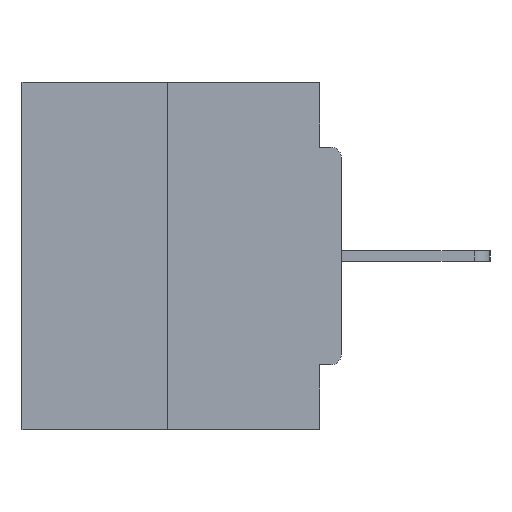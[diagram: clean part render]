
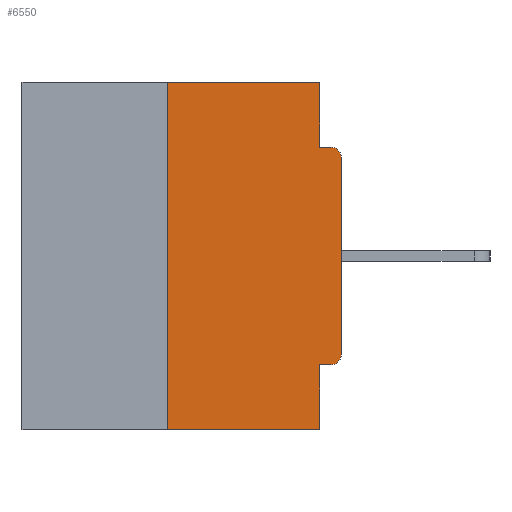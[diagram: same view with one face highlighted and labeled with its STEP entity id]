
A CAD part, left-side view. The second image highlights one B-rep face of the part: STEP entity #6550.
In plain terms, the highlighted planar face has unit normal (-1, 0, 0).
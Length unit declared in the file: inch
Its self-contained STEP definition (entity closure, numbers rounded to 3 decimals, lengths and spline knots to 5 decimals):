
#175 = ORIENTED_EDGE ( 'NONE', *, *, #31595, .F. ) ;
#644 = CARTESIAN_POINT ( 'NONE',  ( 0., 0.031, 0. ) ) ;
#915 = CARTESIAN_POINT ( 'NONE',  ( 0., 0., -0.4065 ) ) ;
#1305 = VERTEX_POINT ( 'NONE', #25709 ) ;
#1580 = DIRECTION ( 'NONE',  ( 0., -1., 0. ) ) ;
#2088 = CARTESIAN_POINT ( 'NONE',  ( 0., 0.031, 0. ) ) ;
#2983 = ORIENTED_EDGE ( 'NONE', *, *, #23573, .F. ) ;
#3215 = EDGE_CURVE ( 'NONE', #24187, #14221, #26456, .T. ) ;
#3456 = VERTEX_POINT ( 'NONE', #5786 ) ;
#3490 = VECTOR ( 'NONE', #1580, 39.37008 ) ;
#3898 = CARTESIAN_POINT ( 'NONE',  ( 0., 0.015, -0.3915 ) ) ;
#3911 = ORIENTED_EDGE ( 'NONE', *, *, #20447, .T. ) ;
#4279 = DIRECTION ( 'NONE',  ( 0., 0., 1. ) ) ;
#4697 = LINE ( 'NONE', #24977, #11802 ) ;
#4890 = EDGE_LOOP ( 'NONE', ( #21691, #175, #27476, #16226, #2983, #3911, #17752, #12775, #15443, #9832 ) ) ;
#5073 = CARTESIAN_POINT ( 'NONE',  ( 0., 0.46, -0.5 ) ) ;
#5786 = CARTESIAN_POINT ( 'NONE',  ( 0., 0.031, -0.0935 ) ) ;
#5982 = LINE ( 'NONE', #6297, #25181 ) ;
#6297 = CARTESIAN_POINT ( 'NONE',  ( 0., 0., 0. ) ) ;
#6550 = ADVANCED_FACE ( 'NONE', ( #20628 ), #17997, .F. ) ;
#7483 = VERTEX_POINT ( 'NONE', #8273 ) ;
#8273 = CARTESIAN_POINT ( 'NONE',  ( 0., 0.25, -0.5 ) ) ;
#8422 = DIRECTION ( 'NONE',  ( 0., 1., 0. ) ) ;
#9832 = ORIENTED_EDGE ( 'NONE', *, *, #13114, .F. ) ;
#9934 = DIRECTION ( 'NONE',  ( 0., -1., 0. ) ) ;
#10700 = AXIS2_PLACEMENT_3D ( 'NONE', #14716, #11786, #19805 ) ;
#10966 = CARTESIAN_POINT ( 'NONE',  ( 0., 0.031, -0.5 ) ) ;
#11416 = DIRECTION ( 'NONE',  ( 0., 0., -1. ) ) ;
#11463 = VECTOR ( 'NONE', #16499, 39.37008 ) ;
#11465 = AXIS2_PLACEMENT_3D ( 'NONE', #3898, #23858, #11416 ) ;
#11786 = DIRECTION ( 'NONE',  ( -1., 0., 0. ) ) ;
#11802 = VECTOR ( 'NONE', #9934, 39.37008 ) ;
#11882 = EDGE_CURVE ( 'NONE', #22223, #21910, #5982, .T. ) ;
#12775 = ORIENTED_EDGE ( 'NONE', *, *, #25974, .T. ) ;
#13114 = EDGE_CURVE ( 'NONE', #14221, #3456, #13359, .T. ) ;
#13236 = LINE ( 'NONE', #10966, #11463 ) ;
#13359 = LINE ( 'NONE', #644, #14504 ) ;
#13407 = CARTESIAN_POINT ( 'NONE',  ( 0., 0.031, -0.5 ) ) ;
#13539 = CIRCLE ( 'NONE', #11465, 0.015 ) ;
#14221 = VERTEX_POINT ( 'NONE', #2088 ) ;
#14504 = VECTOR ( 'NONE', #20743, 39.37008 ) ;
#14716 = CARTESIAN_POINT ( 'NONE',  ( 0., 0.015, -0.1085 ) ) ;
#15443 = ORIENTED_EDGE ( 'NONE', *, *, #32128, .F. ) ;
#15498 = DIRECTION ( 'NONE',  ( 0., -1., 0. ) ) ;
#15654 = LINE ( 'NONE', #5073, #25097 ) ;
#15689 = DIRECTION ( 'NONE',  ( 1., 0., 0. ) ) ;
#16140 = AXIS2_PLACEMENT_3D ( 'NONE', #28148, #15689, #30600 ) ;
#16226 = ORIENTED_EDGE ( 'NONE', *, *, #18710, .F. ) ;
#16408 = VERTEX_POINT ( 'NONE', #13407 ) ;
#16467 = CARTESIAN_POINT ( 'NONE',  ( 0., 0.015, -0.4065 ) ) ;
#16499 = DIRECTION ( 'NONE',  ( 0., 0., -1. ) ) ;
#16653 = CARTESIAN_POINT ( 'NONE',  ( 0., 0.25, 0. ) ) ;
#17752 = ORIENTED_EDGE ( 'NONE', *, *, #11882, .T. ) ;
#17997 = PLANE ( 'NONE',  #16140 ) ;
#18710 = EDGE_CURVE ( 'NONE', #1305, #16408, #13236, .T. ) ;
#19003 = VECTOR ( 'NONE', #8422, 39.37008 ) ;
#19028 = EDGE_CURVE ( 'NONE', #7483, #16408, #15654, .T. ) ;
#19040 = CARTESIAN_POINT ( 'NONE',  ( 0., 0., -0.1085 ) ) ;
#19182 = VERTEX_POINT ( 'NONE', #16467 ) ;
#19805 = DIRECTION ( 'NONE',  ( 0., 0., -1. ) ) ;
#20447 = EDGE_CURVE ( 'NONE', #19182, #22223, #13539, .T. ) ;
#20628 = FACE_OUTER_BOUND ( 'NONE', #4890, .T. ) ;
#20743 = DIRECTION ( 'NONE',  ( 0., 0., -1. ) ) ;
#21138 = CARTESIAN_POINT ( 'NONE',  ( 0., 0.25, 0. ) ) ;
#21691 = ORIENTED_EDGE ( 'NONE', *, *, #3215, .F. ) ;
#21910 = VERTEX_POINT ( 'NONE', #19040 ) ;
#22223 = VERTEX_POINT ( 'NONE', #28182 ) ;
#23573 = EDGE_CURVE ( 'NONE', #19182, #1305, #26087, .T. ) ;
#23744 = VERTEX_POINT ( 'NONE', #31915 ) ;
#23858 = DIRECTION ( 'NONE',  ( -1., 0., 0. ) ) ;
#23984 = CARTESIAN_POINT ( 'NONE',  ( 0., 0.46, 0. ) ) ;
#24077 = LINE ( 'NONE', #21138, #31096 ) ;
#24187 = VERTEX_POINT ( 'NONE', #16653 ) ;
#24977 = CARTESIAN_POINT ( 'NONE',  ( 0., 0., -0.0935 ) ) ;
#25097 = VECTOR ( 'NONE', #15498, 39.37008 ) ;
#25181 = VECTOR ( 'NONE', #31006, 39.37008 ) ;
#25709 = CARTESIAN_POINT ( 'NONE',  ( 0., 0.031, -0.4065 ) ) ;
#25974 = EDGE_CURVE ( 'NONE', #21910, #23744, #26891, .T. ) ;
#26087 = LINE ( 'NONE', #915, #19003 ) ;
#26456 = LINE ( 'NONE', #23984, #3490 ) ;
#26891 = CIRCLE ( 'NONE', #10700, 0.015 ) ;
#27476 = ORIENTED_EDGE ( 'NONE', *, *, #19028, .T. ) ;
#28148 = CARTESIAN_POINT ( 'NONE',  ( 0., 0.46, 0. ) ) ;
#28182 = CARTESIAN_POINT ( 'NONE',  ( 0., 0., -0.3915 ) ) ;
#30600 = DIRECTION ( 'NONE',  ( 0., 0., -1. ) ) ;
#31006 = DIRECTION ( 'NONE',  ( 0., 0., 1. ) ) ;
#31096 = VECTOR ( 'NONE', #4279, 39.37008 ) ;
#31595 = EDGE_CURVE ( 'NONE', #7483, #24187, #24077, .T. ) ;
#31915 = CARTESIAN_POINT ( 'NONE',  ( 0., 0.015, -0.0935 ) ) ;
#32128 = EDGE_CURVE ( 'NONE', #3456, #23744, #4697, .T. ) ;
